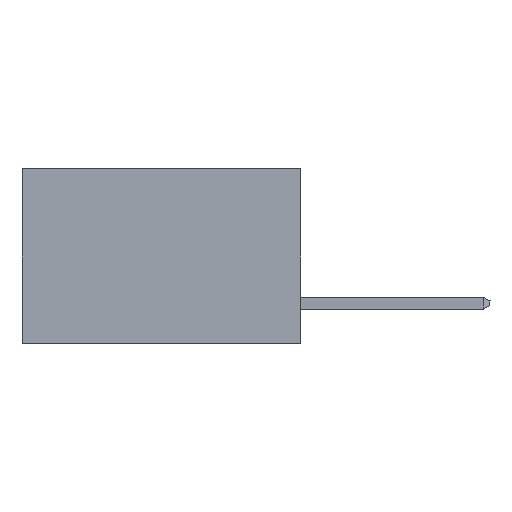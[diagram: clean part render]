
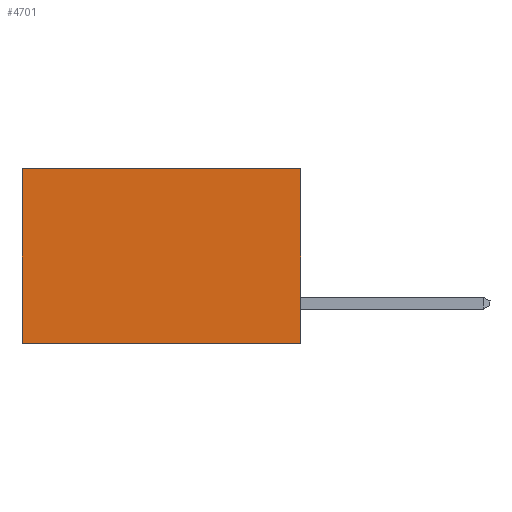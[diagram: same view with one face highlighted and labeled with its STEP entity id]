
A CAD part, left-side view. The second image highlights one B-rep face of the part: STEP entity #4701.
In plain terms, the highlighted planar face has unit normal (-1, 0, 0).
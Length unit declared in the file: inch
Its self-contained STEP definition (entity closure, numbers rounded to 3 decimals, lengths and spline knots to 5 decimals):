
#168 = CARTESIAN_POINT ( 'NONE',  ( 0.277, 0., -0.37 ) ) ;
#808 = EDGE_CURVE ( 'NONE', #10597, #11519, #9483, .T. ) ;
#1910 = CARTESIAN_POINT ( 'NONE',  ( 0.277, 0.59, -0.37 ) ) ;
#2149 = CARTESIAN_POINT ( 'NONE',  ( 0.277, 0., -0.37 ) ) ;
#2342 = DIRECTION ( 'NONE',  ( 0., 0., -1. ) ) ;
#2697 = DIRECTION ( 'NONE',  ( 0., 0., -1. ) ) ;
#2766 = EDGE_CURVE ( 'NONE', #10597, #8151, #9853, .T. ) ;
#2768 = ORIENTED_EDGE ( 'NONE', *, *, #7093, .F. ) ;
#3323 = FACE_OUTER_BOUND ( 'NONE', #7583, .T. ) ;
#3656 = CARTESIAN_POINT ( 'NONE',  ( 0.277, 0.59, 0. ) ) ;
#4701 = ADVANCED_FACE ( 'NONE', ( #3323 ), #9726, .F. ) ;
#4852 = CARTESIAN_POINT ( 'NONE',  ( 0.277, 0., 0. ) ) ;
#5305 = VERTEX_POINT ( 'NONE', #1910 ) ;
#5610 = ORIENTED_EDGE ( 'NONE', *, *, #2766, .F. ) ;
#5775 = CARTESIAN_POINT ( 'NONE',  ( 0.277, 0., -0.37 ) ) ;
#5786 = DIRECTION ( 'NONE',  ( 0., 1., 0. ) ) ;
#6152 = LINE ( 'NONE', #9928, #10779 ) ;
#6866 = VECTOR ( 'NONE', #7176, 39.37008 ) ;
#7093 = EDGE_CURVE ( 'NONE', #8151, #5305, #12412, .T. ) ;
#7176 = DIRECTION ( 'NONE',  ( 0., 1., 0. ) ) ;
#7583 = EDGE_LOOP ( 'NONE', ( #10616, #2768, #5610, #10936 ) ) ;
#8151 = VERTEX_POINT ( 'NONE', #5775 ) ;
#9405 = DIRECTION ( 'NONE',  ( 0., 0., -1. ) ) ;
#9407 = DIRECTION ( 'NONE',  ( 1., 0., 0. ) ) ;
#9483 = LINE ( 'NONE', #11940, #6866 ) ;
#9587 = CARTESIAN_POINT ( 'NONE',  ( 0.277, 0., -0.37 ) ) ;
#9726 = PLANE ( 'NONE',  #12327 ) ;
#9794 = VECTOR ( 'NONE', #5786, 39.37008 ) ;
#9853 = LINE ( 'NONE', #2149, #12167 ) ;
#9916 = EDGE_CURVE ( 'NONE', #11519, #5305, #6152, .T. ) ;
#9928 = CARTESIAN_POINT ( 'NONE',  ( 0.277, 0.59, -0.37 ) ) ;
#10597 = VERTEX_POINT ( 'NONE', #4852 ) ;
#10616 = ORIENTED_EDGE ( 'NONE', *, *, #9916, .T. ) ;
#10779 = VECTOR ( 'NONE', #2697, 39.37008 ) ;
#10936 = ORIENTED_EDGE ( 'NONE', *, *, #808, .T. ) ;
#11519 = VERTEX_POINT ( 'NONE', #3656 ) ;
#11940 = CARTESIAN_POINT ( 'NONE',  ( 0.277, 0., 0. ) ) ;
#12167 = VECTOR ( 'NONE', #2342, 39.37008 ) ;
#12327 = AXIS2_PLACEMENT_3D ( 'NONE', #9587, #9407, #9405 ) ;
#12412 = LINE ( 'NONE', #168, #9794 ) ;
